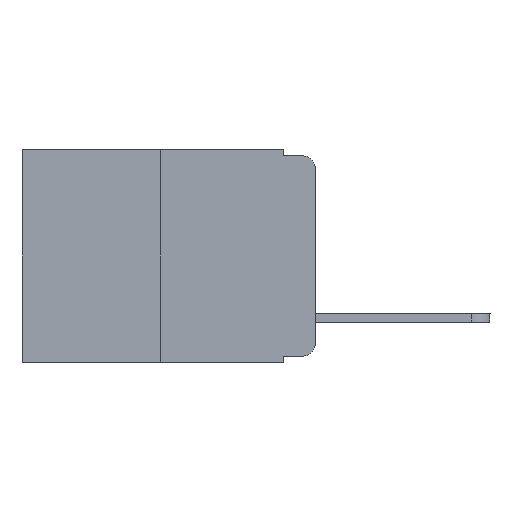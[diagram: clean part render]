
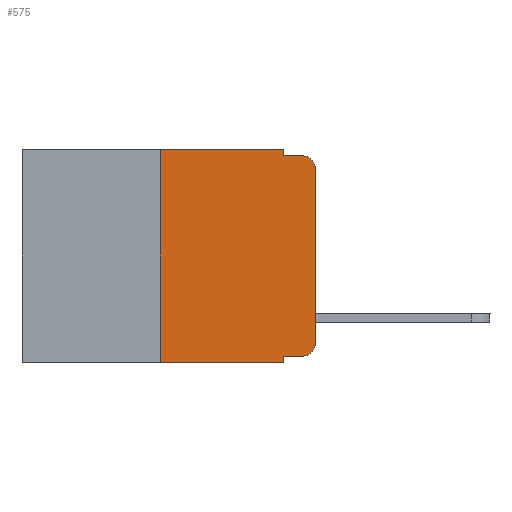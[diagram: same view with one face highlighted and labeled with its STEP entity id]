
A CAD part, left-side view. The second image highlights one B-rep face of the part: STEP entity #575.
In plain terms, the highlighted planar face has unit normal (-1, 0, 0).
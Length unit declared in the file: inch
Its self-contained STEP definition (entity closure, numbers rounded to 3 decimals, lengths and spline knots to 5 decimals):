
#319 = ORIENTED_EDGE ( 'NONE', *, *, #11378, .T. ) ;
#321 = DIRECTION ( 'NONE',  ( 0., 0., 1. ) ) ;
#518 = DIRECTION ( 'NONE',  ( 0., 0., -1. ) ) ;
#575 = ADVANCED_FACE ( 'NONE', ( #10054 ), #3831, .F. ) ;
#903 = CARTESIAN_POINT ( 'NONE',  ( 0., 0.25, -0.343 ) ) ;
#1388 = DIRECTION ( 'NONE',  ( 0., -1., 0. ) ) ;
#1512 = LINE ( 'NONE', #4722, #5804 ) ;
#1820 = CARTESIAN_POINT ( 'NONE',  ( 0., 0.25, 0. ) ) ;
#2355 = LINE ( 'NONE', #19505, #15712 ) ;
#2810 = EDGE_LOOP ( 'NONE', ( #319, #12527, #7858, #9861, #7961, #10582, #11204, #14368, #6382, #18693 ) ) ;
#2878 = DIRECTION ( 'NONE',  ( 0., 0., -1. ) ) ;
#3057 = CARTESIAN_POINT ( 'NONE',  ( 0., 0.02, -0.01 ) ) ;
#3278 = CIRCLE ( 'NONE', #5833, 0.02 ) ;
#3363 = CARTESIAN_POINT ( 'NONE',  ( 0., 0.051, -0.01 ) ) ;
#3548 = DIRECTION ( 'NONE',  ( -1., 0., 0. ) ) ;
#3554 = VECTOR ( 'NONE', #6685, 39.37008 ) ;
#3746 = LINE ( 'NONE', #6746, #11478 ) ;
#3763 = EDGE_CURVE ( 'NONE', #16392, #10340, #3746, .T. ) ;
#3781 = CARTESIAN_POINT ( 'NONE',  ( 0., 0.051, 0. ) ) ;
#3831 = PLANE ( 'NONE',  #18331 ) ;
#4001 = EDGE_CURVE ( 'NONE', #12232, #13969, #10663, .T. ) ;
#4158 = CARTESIAN_POINT ( 'NONE',  ( 0., 0., -0.03 ) ) ;
#4187 = CARTESIAN_POINT ( 'NONE',  ( 0., 0.02, -0.313 ) ) ;
#4722 = CARTESIAN_POINT ( 'NONE',  ( 0., 0.051, -0.01 ) ) ;
#5519 = LINE ( 'NONE', #19559, #13649 ) ;
#5717 = VERTEX_POINT ( 'NONE', #12140 ) ;
#5742 = DIRECTION ( 'NONE',  ( 0., 0., 1. ) ) ;
#5768 = EDGE_CURVE ( 'NONE', #16194, #6644, #1512, .T. ) ;
#5804 = VECTOR ( 'NONE', #13733, 39.37008 ) ;
#5833 = AXIS2_PLACEMENT_3D ( 'NONE', #14586, #3548, #19014 ) ;
#6309 = VERTEX_POINT ( 'NONE', #17542 ) ;
#6382 = ORIENTED_EDGE ( 'NONE', *, *, #16787, .T. ) ;
#6644 = VERTEX_POINT ( 'NONE', #3057 ) ;
#6685 = DIRECTION ( 'NONE',  ( 0., 0., -1. ) ) ;
#6746 = CARTESIAN_POINT ( 'NONE',  ( 0., 0.051, 0. ) ) ;
#7301 = LINE ( 'NONE', #19746, #16724 ) ;
#7524 = EDGE_CURVE ( 'NONE', #13969, #5717, #7301, .T. ) ;
#7706 = LINE ( 'NONE', #13823, #15864 ) ;
#7858 = ORIENTED_EDGE ( 'NONE', *, *, #5768, .F. ) ;
#7961 = ORIENTED_EDGE ( 'NONE', *, *, #7524, .F. ) ;
#8171 = EDGE_CURVE ( 'NONE', #18833, #6644, #3278, .T. ) ;
#9082 = EDGE_CURVE ( 'NONE', #5717, #16194, #17548, .T. ) ;
#9861 = ORIENTED_EDGE ( 'NONE', *, *, #9082, .F. ) ;
#9873 = DIRECTION ( 'NONE',  ( 0., 0., -1. ) ) ;
#10045 = DIRECTION ( 'NONE',  ( 0., -1., 0. ) ) ;
#10054 = FACE_OUTER_BOUND ( 'NONE', #2810, .T. ) ;
#10211 = CARTESIAN_POINT ( 'NONE',  ( 0., 0.25, 0. ) ) ;
#10340 = VERTEX_POINT ( 'NONE', #17477 ) ;
#10582 = ORIENTED_EDGE ( 'NONE', *, *, #4001, .F. ) ;
#10663 = LINE ( 'NONE', #1820, #11164 ) ;
#11164 = VECTOR ( 'NONE', #321, 39.37008 ) ;
#11204 = ORIENTED_EDGE ( 'NONE', *, *, #19069, .T. ) ;
#11371 = AXIS2_PLACEMENT_3D ( 'NONE', #4187, #19447, #2878 ) ;
#11378 = EDGE_CURVE ( 'NONE', #15815, #18833, #2355, .T. ) ;
#11478 = VECTOR ( 'NONE', #9873, 39.37008 ) ;
#11549 = CARTESIAN_POINT ( 'NONE',  ( 0., 0.473, 0. ) ) ;
#12140 = CARTESIAN_POINT ( 'NONE',  ( 0., 0.051, 0. ) ) ;
#12232 = VERTEX_POINT ( 'NONE', #903 ) ;
#12527 = ORIENTED_EDGE ( 'NONE', *, *, #8171, .T. ) ;
#13649 = VECTOR ( 'NONE', #10045, 39.37008 ) ;
#13733 = DIRECTION ( 'NONE',  ( 0., -1., 0. ) ) ;
#13823 = CARTESIAN_POINT ( 'NONE',  ( 0., 0.473, -0.343 ) ) ;
#13969 = VERTEX_POINT ( 'NONE', #10211 ) ;
#14368 = ORIENTED_EDGE ( 'NONE', *, *, #3763, .F. ) ;
#14586 = CARTESIAN_POINT ( 'NONE',  ( 0., 0.02, -0.03 ) ) ;
#15551 = CIRCLE ( 'NONE', #11371, 0.02 ) ;
#15712 = VECTOR ( 'NONE', #5742, 39.37008 ) ;
#15815 = VERTEX_POINT ( 'NONE', #17454 ) ;
#15864 = VECTOR ( 'NONE', #18065, 39.37008 ) ;
#15979 = DIRECTION ( 'NONE',  ( 1., 0., 0. ) ) ;
#16194 = VERTEX_POINT ( 'NONE', #3363 ) ;
#16392 = VERTEX_POINT ( 'NONE', #19119 ) ;
#16724 = VECTOR ( 'NONE', #1388, 39.37008 ) ;
#16787 = EDGE_CURVE ( 'NONE', #16392, #6309, #5519, .T. ) ;
#17454 = CARTESIAN_POINT ( 'NONE',  ( 0., 0., -0.313 ) ) ;
#17477 = CARTESIAN_POINT ( 'NONE',  ( 0., 0.051, -0.343 ) ) ;
#17542 = CARTESIAN_POINT ( 'NONE',  ( 0., 0.02, -0.333 ) ) ;
#17548 = LINE ( 'NONE', #3781, #3554 ) ;
#18065 = DIRECTION ( 'NONE',  ( 0., -1., 0. ) ) ;
#18331 = AXIS2_PLACEMENT_3D ( 'NONE', #11549, #15979, #518 ) ;
#18693 = ORIENTED_EDGE ( 'NONE', *, *, #19451, .T. ) ;
#18833 = VERTEX_POINT ( 'NONE', #4158 ) ;
#19014 = DIRECTION ( 'NONE',  ( 0., 0., -1. ) ) ;
#19069 = EDGE_CURVE ( 'NONE', #12232, #10340, #7706, .T. ) ;
#19119 = CARTESIAN_POINT ( 'NONE',  ( 0., 0.051, -0.333 ) ) ;
#19447 = DIRECTION ( 'NONE',  ( -1., 0., 0. ) ) ;
#19451 = EDGE_CURVE ( 'NONE', #6309, #15815, #15551, .T. ) ;
#19505 = CARTESIAN_POINT ( 'NONE',  ( 0., 0., 0. ) ) ;
#19559 = CARTESIAN_POINT ( 'NONE',  ( 0., 0.051, -0.333 ) ) ;
#19746 = CARTESIAN_POINT ( 'NONE',  ( 0., 0.473, 0. ) ) ;
